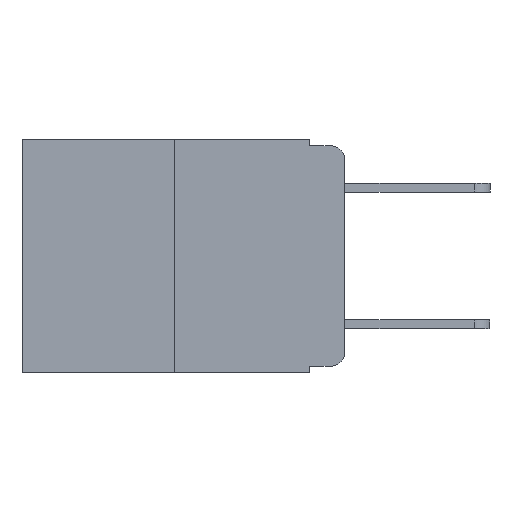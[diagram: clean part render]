
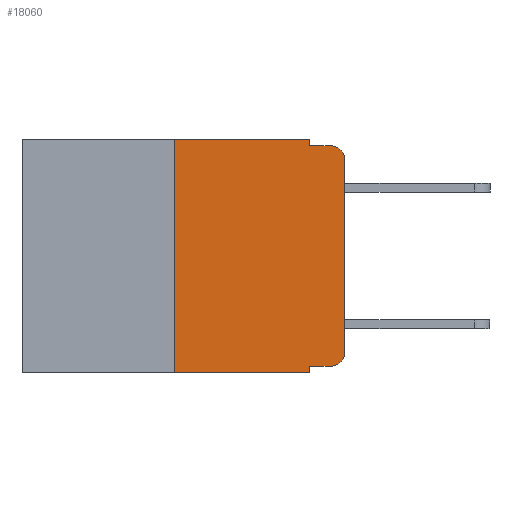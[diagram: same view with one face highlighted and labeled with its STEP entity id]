
A CAD part, left-side view. The second image highlights one B-rep face of the part: STEP entity #18060.
In plain terms, the highlighted planar face has unit normal (-1, 0, 0).
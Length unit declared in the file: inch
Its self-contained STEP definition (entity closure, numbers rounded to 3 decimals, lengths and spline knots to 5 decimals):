
#196 = CARTESIAN_POINT ( 'NONE',  ( 0., 0.051, 0. ) ) ;
#241 = CARTESIAN_POINT ( 'NONE',  ( 0., 0.051, -0.333 ) ) ;
#252 = LINE ( 'NONE', #196, #18920 ) ;
#592 = CARTESIAN_POINT ( 'NONE',  ( 0., 0.051, 0. ) ) ;
#874 = CARTESIAN_POINT ( 'NONE',  ( 0., 0.25, 0. ) ) ;
#1081 = VERTEX_POINT ( 'NONE', #20450 ) ;
#1380 = CARTESIAN_POINT ( 'NONE',  ( 0., 0., -0.313 ) ) ;
#1401 = VECTOR ( 'NONE', #15010, 39.37008 ) ;
#1996 = LINE ( 'NONE', #9577, #1401 ) ;
#2087 = EDGE_CURVE ( 'NONE', #15346, #16379, #20321, .T. ) ;
#2154 = CARTESIAN_POINT ( 'NONE',  ( 0., 0.02, -0.01 ) ) ;
#2155 = DIRECTION ( 'NONE',  ( 0., -1., 0. ) ) ;
#2302 = CARTESIAN_POINT ( 'NONE',  ( 0., 0.473, 0. ) ) ;
#2484 = DIRECTION ( 'NONE',  ( 0., 0., -1. ) ) ;
#2837 = DIRECTION ( 'NONE',  ( -1., 0., 0. ) ) ;
#2870 = CIRCLE ( 'NONE', #22539, 0.02 ) ;
#2873 = ORIENTED_EDGE ( 'NONE', *, *, #2087, .T. ) ;
#3308 = CARTESIAN_POINT ( 'NONE',  ( 0., 0.02, -0.313 ) ) ;
#3347 = EDGE_CURVE ( 'NONE', #11443, #15346, #1996, .T. ) ;
#3379 = ORIENTED_EDGE ( 'NONE', *, *, #20556, .F. ) ;
#3439 = CARTESIAN_POINT ( 'NONE',  ( 0., 0.051, -0.343 ) ) ;
#3828 = CARTESIAN_POINT ( 'NONE',  ( 0., 0.02, -0.03 ) ) ;
#3947 = ORIENTED_EDGE ( 'NONE', *, *, #5571, .T. ) ;
#4163 = ORIENTED_EDGE ( 'NONE', *, *, #22841, .F. ) ;
#4180 = DIRECTION ( 'NONE',  ( 0., 0., -1. ) ) ;
#4462 = DIRECTION ( 'NONE',  ( 0., 0., -1. ) ) ;
#4532 = VERTEX_POINT ( 'NONE', #22162 ) ;
#4538 = VERTEX_POINT ( 'NONE', #18686 ) ;
#4595 = CARTESIAN_POINT ( 'NONE',  ( 0., 0.25, 0. ) ) ;
#5167 = DIRECTION ( 'NONE',  ( 0., 0., -1. ) ) ;
#5571 = EDGE_CURVE ( 'NONE', #8466, #15546, #22544, .T. ) ;
#5787 = ORIENTED_EDGE ( 'NONE', *, *, #19834, .F. ) ;
#5847 = AXIS2_PLACEMENT_3D ( 'NONE', #3828, #2837, #2484 ) ;
#6306 = VECTOR ( 'NONE', #17569, 39.37008 ) ;
#6523 = VECTOR ( 'NONE', #4462, 39.37008 ) ;
#7094 = LINE ( 'NONE', #592, #6523 ) ;
#7139 = CARTESIAN_POINT ( 'NONE',  ( 0., 0.473, -0.343 ) ) ;
#7562 = FACE_OUTER_BOUND ( 'NONE', #20248, .T. ) ;
#7715 = ORIENTED_EDGE ( 'NONE', *, *, #15888, .F. ) ;
#7781 = PLANE ( 'NONE',  #17758 ) ;
#8466 = VERTEX_POINT ( 'NONE', #10247 ) ;
#8510 = VECTOR ( 'NONE', #14354, 39.37008 ) ;
#9577 = CARTESIAN_POINT ( 'NONE',  ( 0., 0., 0. ) ) ;
#9915 = EDGE_CURVE ( 'NONE', #22660, #11443, #2870, .T. ) ;
#10247 = CARTESIAN_POINT ( 'NONE',  ( 0., 0.25, -0.343 ) ) ;
#10652 = DIRECTION ( 'NONE',  ( 0., -1., 0. ) ) ;
#10686 = VERTEX_POINT ( 'NONE', #4595 ) ;
#10784 = LINE ( 'NONE', #241, #19579 ) ;
#11351 = ORIENTED_EDGE ( 'NONE', *, *, #18223, .F. ) ;
#11443 = VERTEX_POINT ( 'NONE', #1380 ) ;
#11878 = DIRECTION ( 'NONE',  ( 0., 0., 1. ) ) ;
#12335 = EDGE_CURVE ( 'NONE', #4538, #22660, #10784, .T. ) ;
#12841 = VECTOR ( 'NONE', #10652, 39.37008 ) ;
#13027 = DIRECTION ( 'NONE',  ( 0., 0., -1. ) ) ;
#13343 = ORIENTED_EDGE ( 'NONE', *, *, #9915, .T. ) ;
#13713 = VECTOR ( 'NONE', #11878, 39.37008 ) ;
#14354 = DIRECTION ( 'NONE',  ( 0., -1., 0. ) ) ;
#14988 = DIRECTION ( 'NONE',  ( 1., 0., 0. ) ) ;
#15010 = DIRECTION ( 'NONE',  ( 0., 0., 1. ) ) ;
#15346 = VERTEX_POINT ( 'NONE', #19017 ) ;
#15546 = VERTEX_POINT ( 'NONE', #3439 ) ;
#15816 = CARTESIAN_POINT ( 'NONE',  ( 0., 0.051, -0.01 ) ) ;
#15888 = EDGE_CURVE ( 'NONE', #4538, #15546, #7094, .T. ) ;
#15925 = DIRECTION ( 'NONE',  ( -1., 0., 0. ) ) ;
#16379 = VERTEX_POINT ( 'NONE', #2154 ) ;
#16958 = LINE ( 'NONE', #19418, #12841 ) ;
#17569 = DIRECTION ( 'NONE',  ( 0., -1., 0. ) ) ;
#17758 = AXIS2_PLACEMENT_3D ( 'NONE', #2302, #14988, #4180 ) ;
#18060 = ADVANCED_FACE ( 'NONE', ( #7562 ), #7781, .F. ) ;
#18223 = EDGE_CURVE ( 'NONE', #8466, #10686, #22443, .T. ) ;
#18686 = CARTESIAN_POINT ( 'NONE',  ( 0., 0.051, -0.333 ) ) ;
#18920 = VECTOR ( 'NONE', #13027, 39.37008 ) ;
#19017 = CARTESIAN_POINT ( 'NONE',  ( 0., 0., -0.03 ) ) ;
#19418 = CARTESIAN_POINT ( 'NONE',  ( 0., 0.473, 0. ) ) ;
#19579 = VECTOR ( 'NONE', #2155, 39.37008 ) ;
#19834 = EDGE_CURVE ( 'NONE', #10686, #1081, #16958, .T. ) ;
#20248 = EDGE_LOOP ( 'NONE', ( #22403, #2873, #4163, #3379, #5787, #11351, #3947, #7715, #22337, #13343 ) ) ;
#20321 = CIRCLE ( 'NONE', #5847, 0.02 ) ;
#20450 = CARTESIAN_POINT ( 'NONE',  ( 0., 0.051, 0. ) ) ;
#20472 = CARTESIAN_POINT ( 'NONE',  ( 0., 0.02, -0.333 ) ) ;
#20485 = LINE ( 'NONE', #15816, #6306 ) ;
#20556 = EDGE_CURVE ( 'NONE', #1081, #4532, #252, .T. ) ;
#22162 = CARTESIAN_POINT ( 'NONE',  ( 0., 0.051, -0.01 ) ) ;
#22337 = ORIENTED_EDGE ( 'NONE', *, *, #12335, .T. ) ;
#22403 = ORIENTED_EDGE ( 'NONE', *, *, #3347, .T. ) ;
#22443 = LINE ( 'NONE', #874, #13713 ) ;
#22539 = AXIS2_PLACEMENT_3D ( 'NONE', #3308, #15925, #5167 ) ;
#22544 = LINE ( 'NONE', #7139, #8510 ) ;
#22660 = VERTEX_POINT ( 'NONE', #20472 ) ;
#22841 = EDGE_CURVE ( 'NONE', #4532, #16379, #20485, .T. ) ;
